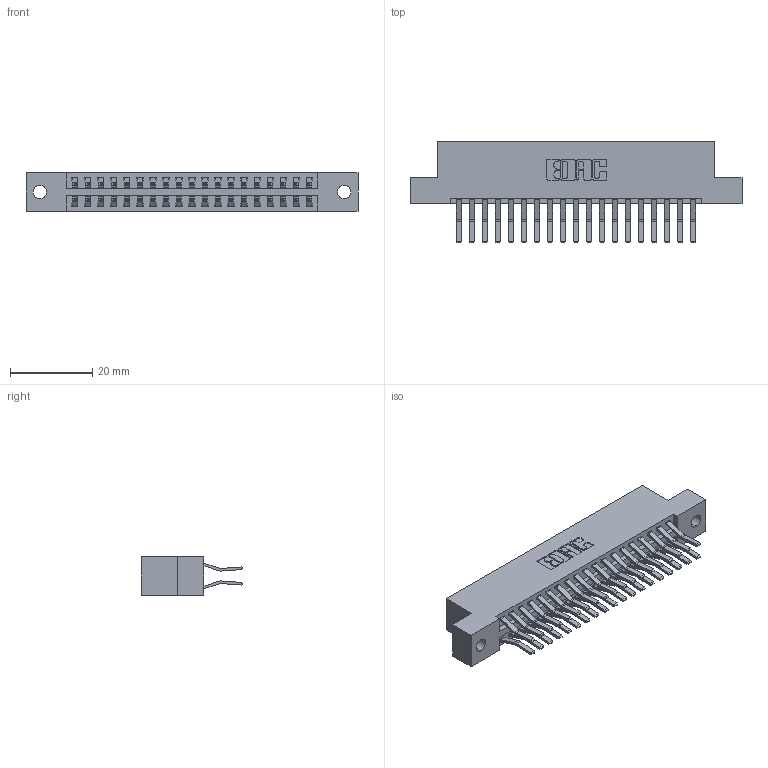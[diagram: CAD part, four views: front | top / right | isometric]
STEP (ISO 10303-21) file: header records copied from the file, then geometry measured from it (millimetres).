
FILE_DESCRIPTION (( 'STEP AP203' ), '1' );
FILE_NAME ('346-038-560-202.STEP', '2018-08-24T06:39:22', ( '' ), ( '' ), 'SwSTEP 2.0', 'SolidWorks 2016', '' );
FILE_SCHEMA (( 'CONFIG_CONTROL_DESIGN' ));
Length unit declared in the file: inch
Products named in the file (3): 346 Part_Flush Mounting Lugs - 0.128 Dia; 345-292-001_560 Tail; 346-038-560-202
Assembly tree (39 placements, depth 2):
  346-038-560-202
    346 Part_Flush Mounting Lugs - 0.128 Dia
    345-292-001_560 Tail  x38
Bounding box: 80.9 x 24.78 x 9.4 mm (x, y, z)
Volume: 7922.4 mm3; surface area: 10923.7 mm2
Topology: 39 solids, 39 shells, 2174 faces, 6447 edges, 4246 vertices
Faces by surface type: plane 1406, cylinder 768
Entity records: 15587 total; most frequent: CARTESIAN_POINT 2600, ORIENTED_EDGE 2534, DIRECTION 2347, EDGE_CURVE 1267, LINE 1055, VECTOR 1055, VERTEX_POINT 842, AXIS2_PLACEMENT_3D 646
